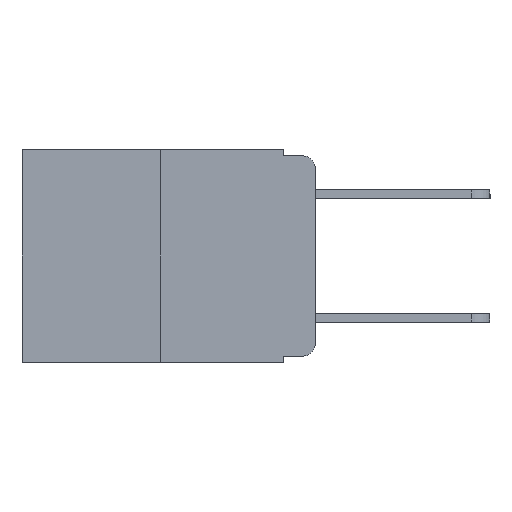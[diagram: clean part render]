
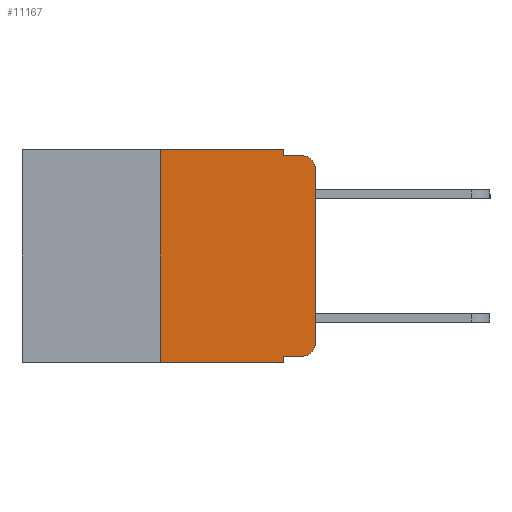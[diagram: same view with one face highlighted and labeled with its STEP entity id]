
A CAD part, left-side view. The second image highlights one B-rep face of the part: STEP entity #11167.
In plain terms, the highlighted planar face has unit normal (-1, 0, 0).
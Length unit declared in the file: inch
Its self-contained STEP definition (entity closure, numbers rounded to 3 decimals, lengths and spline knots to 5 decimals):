
#304 = CARTESIAN_POINT ( 'NONE',  ( 0., 0.25, 0. ) ) ;
#368 = ORIENTED_EDGE ( 'NONE', *, *, #17734, .F. ) ;
#605 = CARTESIAN_POINT ( 'NONE',  ( 0., 0., -0.03 ) ) ;
#1055 = DIRECTION ( 'NONE',  ( 0., 0., -1. ) ) ;
#1290 = EDGE_LOOP ( 'NONE', ( #4535, #5953, #368, #5635, #6307, #14013, #3060, #6329, #5359, #17682 ) ) ;
#1908 = CARTESIAN_POINT ( 'NONE',  ( 0., 0.25, 0. ) ) ;
#2104 = VERTEX_POINT ( 'NONE', #5510 ) ;
#2264 = EDGE_CURVE ( 'NONE', #4032, #11423, #16323, .T. ) ;
#2512 = DIRECTION ( 'NONE',  ( 0., 0., -1. ) ) ;
#2618 = DIRECTION ( 'NONE',  ( 0., 0., -1. ) ) ;
#2656 = VECTOR ( 'NONE', #14776, 39.37008 ) ;
#2899 = CARTESIAN_POINT ( 'NONE',  ( 0., 0.051, 0. ) ) ;
#3060 = ORIENTED_EDGE ( 'NONE', *, *, #14901, .T. ) ;
#3251 = VERTEX_POINT ( 'NONE', #304 ) ;
#3318 = CARTESIAN_POINT ( 'NONE',  ( 0., 0.02, -0.03 ) ) ;
#3429 = VERTEX_POINT ( 'NONE', #8269 ) ;
#3509 = AXIS2_PLACEMENT_3D ( 'NONE', #10477, #22927, #12306 ) ;
#3743 = LINE ( 'NONE', #20612, #12953 ) ;
#4032 = VERTEX_POINT ( 'NONE', #605 ) ;
#4163 = DIRECTION ( 'NONE',  ( 0., -1., 0. ) ) ;
#4535 = ORIENTED_EDGE ( 'NONE', *, *, #6486, .T. ) ;
#5134 = LINE ( 'NONE', #2899, #19054 ) ;
#5144 = DIRECTION ( 'NONE',  ( 0., -1., 0. ) ) ;
#5359 = ORIENTED_EDGE ( 'NONE', *, *, #13567, .T. ) ;
#5475 = CARTESIAN_POINT ( 'NONE',  ( 0., 0.051, -0.01 ) ) ;
#5510 = CARTESIAN_POINT ( 'NONE',  ( 0., 0., -0.313 ) ) ;
#5635 = ORIENTED_EDGE ( 'NONE', *, *, #5858, .F. ) ;
#5858 = EDGE_CURVE ( 'NONE', #3429, #14878, #5134, .T. ) ;
#5953 = ORIENTED_EDGE ( 'NONE', *, *, #2264, .T. ) ;
#5976 = CARTESIAN_POINT ( 'NONE',  ( 0., 0.02, -0.01 ) ) ;
#6106 = CARTESIAN_POINT ( 'NONE',  ( 0., 0.25, -0.343 ) ) ;
#6110 = DIRECTION ( 'NONE',  ( 0., -1., 0. ) ) ;
#6307 = ORIENTED_EDGE ( 'NONE', *, *, #12157, .F. ) ;
#6329 = ORIENTED_EDGE ( 'NONE', *, *, #12780, .F. ) ;
#6486 = EDGE_CURVE ( 'NONE', #2104, #4032, #11471, .T. ) ;
#6501 = CIRCLE ( 'NONE', #3509, 0.02 ) ;
#6527 = CARTESIAN_POINT ( 'NONE',  ( 0., 0., 0. ) ) ;
#6583 = VECTOR ( 'NONE', #22685, 39.37008 ) ;
#7278 = VECTOR ( 'NONE', #16453, 39.37008 ) ;
#7448 = DIRECTION ( 'NONE',  ( -1., 0., 0. ) ) ;
#7856 = LINE ( 'NONE', #15305, #17481 ) ;
#8269 = CARTESIAN_POINT ( 'NONE',  ( 0., 0.051, 0. ) ) ;
#9442 = EDGE_CURVE ( 'NONE', #10694, #2104, #6501, .T. ) ;
#9654 = CARTESIAN_POINT ( 'NONE',  ( 0., 0.051, -0.01 ) ) ;
#9871 = CARTESIAN_POINT ( 'NONE',  ( 0., 0.051, -0.333 ) ) ;
#10006 = PLANE ( 'NONE',  #14322 ) ;
#10477 = CARTESIAN_POINT ( 'NONE',  ( 0., 0.02, -0.313 ) ) ;
#10694 = VERTEX_POINT ( 'NONE', #12099 ) ;
#10924 = VECTOR ( 'NONE', #5144, 39.37008 ) ;
#11167 = ADVANCED_FACE ( 'NONE', ( #18613 ), #10006, .F. ) ;
#11415 = VERTEX_POINT ( 'NONE', #16796 ) ;
#11423 = VERTEX_POINT ( 'NONE', #5976 ) ;
#11471 = LINE ( 'NONE', #6527, #6583 ) ;
#12099 = CARTESIAN_POINT ( 'NONE',  ( 0., 0.02, -0.333 ) ) ;
#12157 = EDGE_CURVE ( 'NONE', #3251, #3429, #7856, .T. ) ;
#12165 = LINE ( 'NONE', #21685, #7278 ) ;
#12306 = DIRECTION ( 'NONE',  ( 0., 0., -1. ) ) ;
#12780 = EDGE_CURVE ( 'NONE', #20388, #11415, #3743, .T. ) ;
#12953 = VECTOR ( 'NONE', #2512, 39.37008 ) ;
#13567 = EDGE_CURVE ( 'NONE', #20388, #10694, #15733, .T. ) ;
#13659 = DIRECTION ( 'NONE',  ( 1., 0., 0. ) ) ;
#14013 = ORIENTED_EDGE ( 'NONE', *, *, #21536, .F. ) ;
#14322 = AXIS2_PLACEMENT_3D ( 'NONE', #22459, #13659, #2618 ) ;
#14776 = DIRECTION ( 'NONE',  ( 0., 0., 1. ) ) ;
#14878 = VERTEX_POINT ( 'NONE', #5475 ) ;
#14901 = EDGE_CURVE ( 'NONE', #15615, #11415, #12165, .T. ) ;
#15054 = DIRECTION ( 'NONE',  ( 0., 0., -1. ) ) ;
#15305 = CARTESIAN_POINT ( 'NONE',  ( 0., 0.473, 0. ) ) ;
#15615 = VERTEX_POINT ( 'NONE', #6106 ) ;
#15733 = LINE ( 'NONE', #17872, #10924 ) ;
#16323 = CIRCLE ( 'NONE', #21279, 0.02 ) ;
#16453 = DIRECTION ( 'NONE',  ( 0., -1., 0. ) ) ;
#16796 = CARTESIAN_POINT ( 'NONE',  ( 0., 0.051, -0.343 ) ) ;
#17063 = LINE ( 'NONE', #9654, #21193 ) ;
#17233 = LINE ( 'NONE', #1908, #2656 ) ;
#17481 = VECTOR ( 'NONE', #6110, 39.37008 ) ;
#17682 = ORIENTED_EDGE ( 'NONE', *, *, #9442, .T. ) ;
#17734 = EDGE_CURVE ( 'NONE', #14878, #11423, #17063, .T. ) ;
#17872 = CARTESIAN_POINT ( 'NONE',  ( 0., 0.051, -0.333 ) ) ;
#18613 = FACE_OUTER_BOUND ( 'NONE', #1290, .T. ) ;
#19054 = VECTOR ( 'NONE', #1055, 39.37008 ) ;
#20388 = VERTEX_POINT ( 'NONE', #9871 ) ;
#20612 = CARTESIAN_POINT ( 'NONE',  ( 0., 0.051, 0. ) ) ;
#21193 = VECTOR ( 'NONE', #4163, 39.37008 ) ;
#21279 = AXIS2_PLACEMENT_3D ( 'NONE', #3318, #7448, #15054 ) ;
#21536 = EDGE_CURVE ( 'NONE', #15615, #3251, #17233, .T. ) ;
#21685 = CARTESIAN_POINT ( 'NONE',  ( 0., 0.473, -0.343 ) ) ;
#22459 = CARTESIAN_POINT ( 'NONE',  ( 0., 0.473, 0. ) ) ;
#22685 = DIRECTION ( 'NONE',  ( 0., 0., 1. ) ) ;
#22927 = DIRECTION ( 'NONE',  ( -1., 0., 0. ) ) ;
